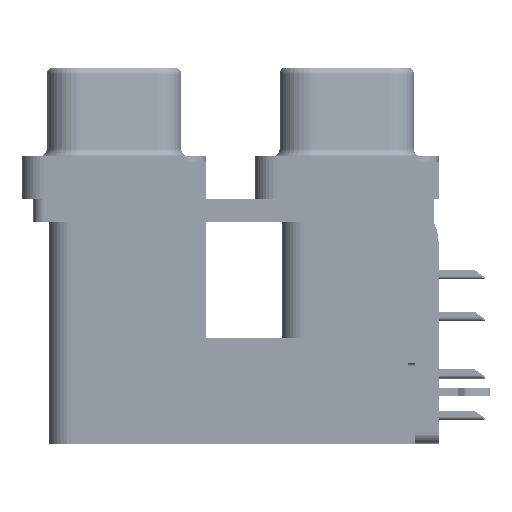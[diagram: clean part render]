
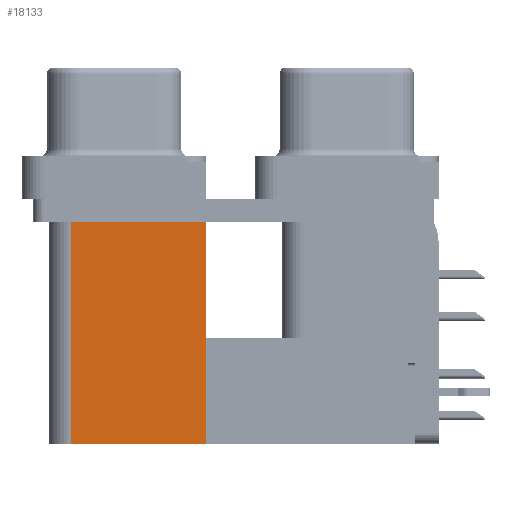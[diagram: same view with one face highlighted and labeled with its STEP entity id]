
A CAD part, left-side view. The second image highlights one B-rep face of the part: STEP entity #18133.
In plain terms, the highlighted planar face has unit normal (-1, 0, 0).
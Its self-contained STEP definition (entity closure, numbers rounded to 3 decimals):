
#3245 = CARTESIAN_POINT ( 'NONE',  ( 3.79, 18.8, -19.2 ) ) ;
#6027 = ORIENTED_EDGE ( 'NONE', *, *, #17199, .T. ) ;
#6218 = LINE ( 'NONE', #6750, #18901 ) ;
#6664 = AXIS2_PLACEMENT_3D ( 'NONE', #12018, #20296, #11759 ) ;
#6750 = CARTESIAN_POINT ( 'NONE',  ( 3.79, 9.6, -19.2 ) ) ;
#9873 = CARTESIAN_POINT ( 'NONE',  ( 3.79, 18.8, -19.2 ) ) ;
#11759 = DIRECTION ( 'NONE',  ( 0., 0., -1. ) ) ;
#12018 = CARTESIAN_POINT ( 'NONE',  ( 3.79, 9.6, -19.2 ) ) ;
#13829 = CARTESIAN_POINT ( 'NONE',  ( 3.79, 18.8, -2.5 ) ) ;
#16490 = EDGE_CURVE ( 'NONE', #26172, #42572, #33052, .T. ) ;
#16844 = ORIENTED_EDGE ( 'NONE', *, *, #21233, .F. ) ;
#17199 = EDGE_CURVE ( 'NONE', #39031, #26172, #24496, .T. ) ;
#17760 = CARTESIAN_POINT ( 'NONE',  ( 3.79, 9.6, -2.5 ) ) ;
#18133 = ADVANCED_FACE ( 'NONE', ( #38997 ), #44321, .F. ) ;
#18901 = VECTOR ( 'NONE', #31007, 1000. ) ;
#20296 = DIRECTION ( 'NONE',  ( 1., 0., 0. ) ) ;
#21233 = EDGE_CURVE ( 'NONE', #39031, #28487, #6218, .T. ) ;
#21955 = CARTESIAN_POINT ( 'NONE',  ( 3.79, 9.6, -19.2 ) ) ;
#24496 = LINE ( 'NONE', #36487, #30424 ) ;
#26172 = VERTEX_POINT ( 'NONE', #17760 ) ;
#26777 = ORIENTED_EDGE ( 'NONE', *, *, #50746, .F. ) ;
#27275 = DIRECTION ( 'NONE',  ( 0., 0., 1. ) ) ;
#28487 = VERTEX_POINT ( 'NONE', #3245 ) ;
#30424 = VECTOR ( 'NONE', #27275, 1000. ) ;
#30926 = LINE ( 'NONE', #9873, #34574 ) ;
#31007 = DIRECTION ( 'NONE',  ( 0., 1., 0. ) ) ;
#33052 = LINE ( 'NONE', #41077, #41482 ) ;
#34574 = VECTOR ( 'NONE', #38427, 1000. ) ;
#35205 = EDGE_LOOP ( 'NONE', ( #43518, #26777, #16844, #6027 ) ) ;
#36487 = CARTESIAN_POINT ( 'NONE',  ( 3.79, 9.6, -19.2 ) ) ;
#38427 = DIRECTION ( 'NONE',  ( 0., 0., 1. ) ) ;
#38997 = FACE_OUTER_BOUND ( 'NONE', #35205, .T. ) ;
#39031 = VERTEX_POINT ( 'NONE', #21955 ) ;
#41077 = CARTESIAN_POINT ( 'NONE',  ( 3.79, 9.6, -2.5 ) ) ;
#41482 = VECTOR ( 'NONE', #41602, 1000. ) ;
#41602 = DIRECTION ( 'NONE',  ( 0., 1., 0. ) ) ;
#42572 = VERTEX_POINT ( 'NONE', #13829 ) ;
#43518 = ORIENTED_EDGE ( 'NONE', *, *, #16490, .T. ) ;
#44321 = PLANE ( 'NONE',  #6664 ) ;
#50746 = EDGE_CURVE ( 'NONE', #28487, #42572, #30926, .T. ) ;
